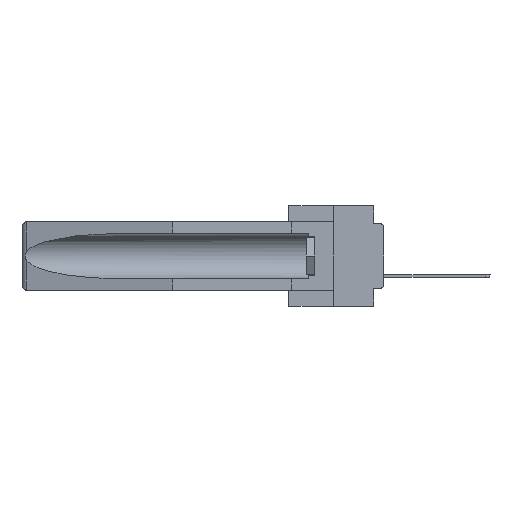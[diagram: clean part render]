
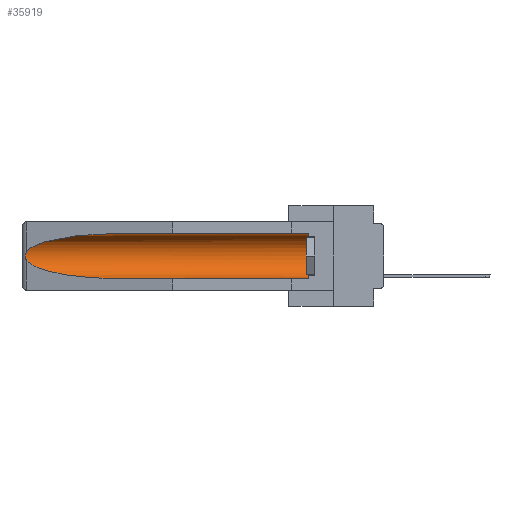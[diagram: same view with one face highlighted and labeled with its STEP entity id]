
A CAD part, left-side view. The second image highlights one B-rep face of the part: STEP entity #35919.
In plain terms, the highlighted cylindrical face has radius 2.857 mm (diameter 5.715 mm), a partial arc.
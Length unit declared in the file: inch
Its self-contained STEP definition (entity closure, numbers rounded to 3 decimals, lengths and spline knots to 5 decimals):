
#73 = CARTESIAN_POINT ( 'NONE',  ( 0.21114, 1.30732, -0.059 ) ) ;
#119 = CARTESIAN_POINT ( 'NONE',  ( 0.155, 0.126, -0.1715 ) ) ;
#1055 = CARTESIAN_POINT ( 'NONE',  ( 0.2673, 1.5327, -0.16383 ) ) ;
#1122 = ORIENTED_EDGE ( 'NONE', *, *, #14699, .T. ) ;
#1168 = CARTESIAN_POINT ( 'NONE',  ( 0.2673, 1.53269, -0.17917 ) ) ;
#1655 = DIRECTION ( 'NONE',  ( 0., 1., 0. ) ) ;
#2074 =( BOUNDED_CURVE ( )  B_SPLINE_CURVE ( 3, ( #36035, #73, #13545, #21988 ),
 .UNSPECIFIED., .F., .F. ) 
 B_SPLINE_CURVE_WITH_KNOTS ( ( 4, 4 ),
 ( 4.71239, 6.08839 ),
 .UNSPECIFIED. ) 
 CURVE ( )  GEOMETRIC_REPRESENTATION_ITEM ( )  RATIONAL_B_SPLINE_CURVE ( ( 1., 0.848, 0.848, 1. ) ) 
 REPRESENTATION_ITEM ( '' )  );
#2444 = ORIENTED_EDGE ( 'NONE', *, *, #24724, .F. ) ;
#4995 = CARTESIAN_POINT ( 'NONE',  ( 0.21114, 1.30732, -0.284 ) ) ;
#5548 = FACE_OUTER_BOUND ( 'NONE', #24702, .T. ) ;
#5839 = B_SPLINE_CURVE_WITH_KNOTS ( 'NONE', 3,
 ( #20982, #9336, #34556, #1055, #20599, #23415, #1168, #6660, #26216, #13167 ),
 .UNSPECIFIED., .F., .F.,
 ( 4, 2, 2, 2, 4 ),
 ( 0., 0.00029, 0.00058, 0.00087, 0.00117 ),
 .UNSPECIFIED. ) ;
#6660 = CARTESIAN_POINT ( 'NONE',  ( 0.26655, 1.53094, -0.18657 ) ) ;
#7663 = VECTOR ( 'NONE', #26244, 39.37008 ) ;
#7721 = LINE ( 'NONE', #31590, #16906 ) ;
#8198 = ORIENTED_EDGE ( 'NONE', *, *, #30149, .T. ) ;
#9336 = CARTESIAN_POINT ( 'NONE',  ( 0.26597, 1.52961, -0.15275 ) ) ;
#9620 = VERTEX_POINT ( 'NONE', #12555 ) ;
#10085 = VERTEX_POINT ( 'NONE', #30247 ) ;
#10386 = CARTESIAN_POINT ( 'NONE',  ( 0.155, 1.07973, -0.284 ) ) ;
#12555 = CARTESIAN_POINT ( 'NONE',  ( 0.155, 1.07973, -0.284 ) ) ;
#13167 = CARTESIAN_POINT ( 'NONE',  ( 0.26537, 1.52718, -0.19328 ) ) ;
#13545 = CARTESIAN_POINT ( 'NONE',  ( 0.25451, 1.48313, -0.09465 ) ) ;
#13884 = CYLINDRICAL_SURFACE ( 'NONE', #20016, 0.1125 ) ;
#14699 = EDGE_CURVE ( 'NONE', #21568, #10085, #5839, .T. ) ;
#15691 = ORIENTED_EDGE ( 'NONE', *, *, #26716, .T. ) ;
#16362 = CARTESIAN_POINT ( 'NONE',  ( 0.26537, 1.52718, -0.19328 ) ) ;
#16724 = CARTESIAN_POINT ( 'NONE',  ( 0.26537, 1.52718, -0.14972 ) ) ;
#16906 = VECTOR ( 'NONE', #1655, 39.37008 ) ;
#17384 = CARTESIAN_POINT ( 'NONE',  ( 0.155, 0.126, -0.059 ) ) ;
#17751 =( BOUNDED_CURVE ( )  B_SPLINE_CURVE ( 3, ( #16362, #27263, #4995, #10386 ),
 .UNSPECIFIED., .F., .F. ) 
 B_SPLINE_CURVE_WITH_KNOTS ( ( 4, 4 ),
 ( 0.1948, 1.5708 ),
 .UNSPECIFIED. ) 
 CURVE ( )  GEOMETRIC_REPRESENTATION_ITEM ( )  RATIONAL_B_SPLINE_CURVE ( ( 1., 0.848, 0.848, 1. ) ) 
 REPRESENTATION_ITEM ( '' )  );
#18370 = CARTESIAN_POINT ( 'NONE',  ( 0.155, -0.30754, -0.1715 ) ) ;
#19384 = CIRCLE ( 'NONE', #30200, 0.1125 ) ;
#19696 = EDGE_CURVE ( 'NONE', #34146, #24861, #19384, .T. ) ;
#20016 = AXIS2_PLACEMENT_3D ( 'NONE', #18370, #27144, #30529 ) ;
#20599 = CARTESIAN_POINT ( 'NONE',  ( 0.2675, 1.53308, -0.16763 ) ) ;
#20880 = CARTESIAN_POINT ( 'NONE',  ( 0.155, -0.30754, -0.284 ) ) ;
#20982 = CARTESIAN_POINT ( 'NONE',  ( 0.26537, 1.52718, -0.14972 ) ) ;
#21403 = VERTEX_POINT ( 'NONE', #25824 ) ;
#21568 = VERTEX_POINT ( 'NONE', #16724 ) ;
#21988 = CARTESIAN_POINT ( 'NONE',  ( 0.26537, 1.52718, -0.14972 ) ) ;
#22824 = EDGE_CURVE ( 'NONE', #24861, #21403, #7721, .T. ) ;
#23383 = CARTESIAN_POINT ( 'NONE',  ( 0.155, 0.126, -0.284 ) ) ;
#23415 = CARTESIAN_POINT ( 'NONE',  ( 0.2675, 1.53308, -0.17534 ) ) ;
#24702 = EDGE_LOOP ( 'NONE', ( #8198, #1122, #15691, #2444, #31204, #35389 ) ) ;
#24724 = EDGE_CURVE ( 'NONE', #34146, #9620, #33063, .T. ) ;
#24861 = VERTEX_POINT ( 'NONE', #17384 ) ;
#25188 = DIRECTION ( 'NONE',  ( 0., -1., 0. ) ) ;
#25409 = DIRECTION ( 'NONE',  ( 0., 0., 1. ) ) ;
#25824 = CARTESIAN_POINT ( 'NONE',  ( 0.155, 1.07973, -0.059 ) ) ;
#26216 = CARTESIAN_POINT ( 'NONE',  ( 0.26597, 1.5296, -0.19026 ) ) ;
#26244 = DIRECTION ( 'NONE',  ( 0., 1., 0. ) ) ;
#26716 = EDGE_CURVE ( 'NONE', #10085, #9620, #17751, .T. ) ;
#27144 = DIRECTION ( 'NONE',  ( 0., 1., 0. ) ) ;
#27263 = CARTESIAN_POINT ( 'NONE',  ( 0.25451, 1.48313, -0.24835 ) ) ;
#30149 = EDGE_CURVE ( 'NONE', #21403, #21568, #2074, .T. ) ;
#30200 = AXIS2_PLACEMENT_3D ( 'NONE', #119, #25188, #25409 ) ;
#30247 = CARTESIAN_POINT ( 'NONE',  ( 0.26537, 1.52718, -0.19328 ) ) ;
#30529 = DIRECTION ( 'NONE',  ( 0., 0., 1. ) ) ;
#31204 = ORIENTED_EDGE ( 'NONE', *, *, #19696, .T. ) ;
#31590 = CARTESIAN_POINT ( 'NONE',  ( 0.155, -0.30754, -0.059 ) ) ;
#33063 = LINE ( 'NONE', #20880, #7663 ) ;
#34146 = VERTEX_POINT ( 'NONE', #23383 ) ;
#34556 = CARTESIAN_POINT ( 'NONE',  ( 0.26654, 1.53092, -0.15636 ) ) ;
#35389 = ORIENTED_EDGE ( 'NONE', *, *, #22824, .T. ) ;
#35919 = ADVANCED_FACE ( 'NONE', ( #5548 ), #13884, .F. ) ;
#36035 = CARTESIAN_POINT ( 'NONE',  ( 0.155, 1.07973, -0.059 ) ) ;
